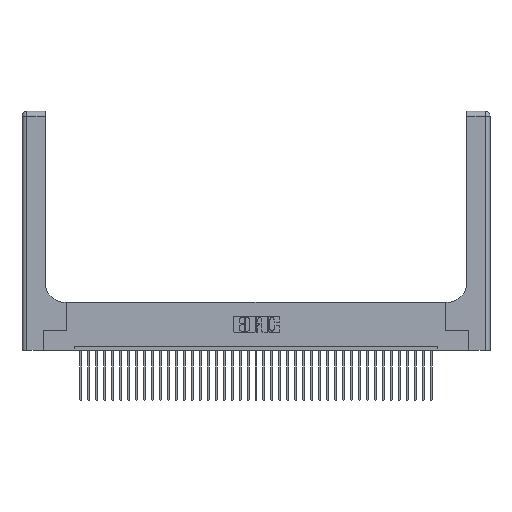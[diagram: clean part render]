
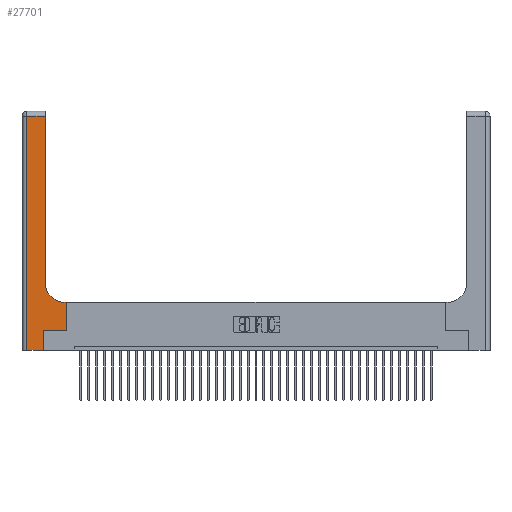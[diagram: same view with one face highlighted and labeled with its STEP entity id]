
A CAD part, top view. The second image highlights one B-rep face of the part: STEP entity #27701.
In plain terms, the highlighted planar face has unit normal (0, 0, 1).
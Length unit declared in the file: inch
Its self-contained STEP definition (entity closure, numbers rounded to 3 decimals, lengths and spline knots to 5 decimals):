
#327 = CARTESIAN_POINT ( 'NONE',  ( 0., 2.94, 0.37 ) ) ;
#449 = ORIENTED_EDGE ( 'NONE', *, *, #11067, .T. ) ;
#457 = CARTESIAN_POINT ( 'NONE',  ( 0.5585, 0.25, 0.37 ) ) ;
#774 = DIRECTION ( 'NONE',  ( 1., 0., 0. ) ) ;
#1066 = EDGE_CURVE ( 'NONE', #9339, #6061, #38326, .T. ) ;
#1150 = EDGE_CURVE ( 'NONE', #20981, #31598, #34036, .T. ) ;
#2347 = CARTESIAN_POINT ( 'NONE',  ( 0.269, 0., 0.37 ) ) ;
#2541 = ORIENTED_EDGE ( 'NONE', *, *, #31981, .T. ) ;
#2677 = CARTESIAN_POINT ( 'NONE',  ( 0.2915, 0.6, 0.37 ) ) ;
#3018 = CARTESIAN_POINT ( 'NONE',  ( 0.06, 2.94, 0.37 ) ) ;
#3461 = CARTESIAN_POINT ( 'NONE',  ( 0.06, 3., 0.37 ) ) ;
#3652 = CARTESIAN_POINT ( 'NONE',  ( 0., 0., 0.37 ) ) ;
#3857 = ORIENTED_EDGE ( 'NONE', *, *, #1150, .T. ) ;
#3983 = CARTESIAN_POINT ( 'NONE',  ( 0., 3., 0.37 ) ) ;
#6061 = VERTEX_POINT ( 'NONE', #13096 ) ;
#6154 = DIRECTION ( 'NONE',  ( 1., 0., 0. ) ) ;
#6666 = EDGE_CURVE ( 'NONE', #35451, #25178, #19521, .T. ) ;
#6714 = DIRECTION ( 'NONE',  ( 0., 1., 0. ) ) ;
#6899 = VECTOR ( 'NONE', #6154, 39.37008 ) ;
#8482 = LINE ( 'NONE', #327, #11281 ) ;
#8506 = VECTOR ( 'NONE', #35838, 39.37008 ) ;
#8776 = LINE ( 'NONE', #16164, #14844 ) ;
#9100 = AXIS2_PLACEMENT_3D ( 'NONE', #26409, #32479, #14501 ) ;
#9339 = VERTEX_POINT ( 'NONE', #3018 ) ;
#10560 = LINE ( 'NONE', #27104, #27389 ) ;
#10849 = ORIENTED_EDGE ( 'NONE', *, *, #1066, .T. ) ;
#11067 = EDGE_CURVE ( 'NONE', #16129, #37402, #10560, .T. ) ;
#11281 = VECTOR ( 'NONE', #27339, 39.37008 ) ;
#12824 = DIRECTION ( 'NONE',  ( -1., 0., 0. ) ) ;
#13096 = CARTESIAN_POINT ( 'NONE',  ( 0.06, 0., 0.37 ) ) ;
#13602 = LINE ( 'NONE', #2677, #8506 ) ;
#14501 = DIRECTION ( 'NONE',  ( 1., 0., 0. ) ) ;
#14844 = VECTOR ( 'NONE', #774, 39.37008 ) ;
#15590 = ORIENTED_EDGE ( 'NONE', *, *, #6666, .T. ) ;
#16129 = VERTEX_POINT ( 'NONE', #32426 ) ;
#16164 = CARTESIAN_POINT ( 'NONE',  ( 0.269, 0.25, 0.37 ) ) ;
#18965 = DIRECTION ( 'NONE',  ( 0., 0., -1. ) ) ;
#19521 = LINE ( 'NONE', #37189, #31771 ) ;
#20481 = AXIS2_PLACEMENT_3D ( 'NONE', #3983, #18965, #12824 ) ;
#20981 = VERTEX_POINT ( 'NONE', #28748 ) ;
#22111 = EDGE_CURVE ( 'NONE', #24100, #16129, #25186, .T. ) ;
#24100 = VERTEX_POINT ( 'NONE', #31450 ) ;
#24358 = EDGE_LOOP ( 'NONE', ( #449, #36393, #10849, #2541, #15590, #25495, #3857, #32150, #36132 ) ) ;
#25178 = VERTEX_POINT ( 'NONE', #25886 ) ;
#25186 = CIRCLE ( 'NONE', #9100, 0.25 ) ;
#25495 = ORIENTED_EDGE ( 'NONE', *, *, #36595, .T. ) ;
#25886 = CARTESIAN_POINT ( 'NONE',  ( 0.269, 0.25, 0.37 ) ) ;
#26409 = CARTESIAN_POINT ( 'NONE',  ( 0.5415, 0.85, 0.37 ) ) ;
#26576 = VECTOR ( 'NONE', #6714, 39.37008 ) ;
#27104 = CARTESIAN_POINT ( 'NONE',  ( 0.2915, 3., 0.37 ) ) ;
#27339 = DIRECTION ( 'NONE',  ( -1., 0., 0. ) ) ;
#27389 = VECTOR ( 'NONE', #32669, 39.37008 ) ;
#27701 = ADVANCED_FACE ( 'NONE', ( #35363 ), #36633, .F. ) ;
#28748 = CARTESIAN_POINT ( 'NONE',  ( 0.5585, 0.25, 0.37 ) ) ;
#28937 = LINE ( 'NONE', #3652, #6899 ) ;
#29884 = VECTOR ( 'NONE', #36261, 39.37008 ) ;
#30015 = EDGE_CURVE ( 'NONE', #31598, #24100, #13602, .T. ) ;
#30981 = DIRECTION ( 'NONE',  ( 0., 1., 0. ) ) ;
#31450 = CARTESIAN_POINT ( 'NONE',  ( 0.5415, 0.6, 0.37 ) ) ;
#31598 = VERTEX_POINT ( 'NONE', #37208 ) ;
#31771 = VECTOR ( 'NONE', #30981, 39.37008 ) ;
#31981 = EDGE_CURVE ( 'NONE', #6061, #35451, #28937, .T. ) ;
#32150 = ORIENTED_EDGE ( 'NONE', *, *, #30015, .T. ) ;
#32426 = CARTESIAN_POINT ( 'NONE',  ( 0.2915, 0.85, 0.37 ) ) ;
#32479 = DIRECTION ( 'NONE',  ( 0., 0., -1. ) ) ;
#32669 = DIRECTION ( 'NONE',  ( 0., 1., 0. ) ) ;
#34036 = LINE ( 'NONE', #457, #26576 ) ;
#34316 = CARTESIAN_POINT ( 'NONE',  ( 0.2915, 2.94, 0.37 ) ) ;
#34459 = EDGE_CURVE ( 'NONE', #37402, #9339, #8482, .T. ) ;
#35363 = FACE_OUTER_BOUND ( 'NONE', #24358, .T. ) ;
#35451 = VERTEX_POINT ( 'NONE', #2347 ) ;
#35838 = DIRECTION ( 'NONE',  ( -1., 0., 0. ) ) ;
#36132 = ORIENTED_EDGE ( 'NONE', *, *, #22111, .T. ) ;
#36261 = DIRECTION ( 'NONE',  ( 0., -1., 0. ) ) ;
#36393 = ORIENTED_EDGE ( 'NONE', *, *, #34459, .T. ) ;
#36595 = EDGE_CURVE ( 'NONE', #25178, #20981, #8776, .T. ) ;
#36633 = PLANE ( 'NONE',  #20481 ) ;
#37189 = CARTESIAN_POINT ( 'NONE',  ( 0.269, 0., 0.37 ) ) ;
#37208 = CARTESIAN_POINT ( 'NONE',  ( 0.5585, 0.6, 0.37 ) ) ;
#37402 = VERTEX_POINT ( 'NONE', #34316 ) ;
#38326 = LINE ( 'NONE', #3461, #29884 ) ;
